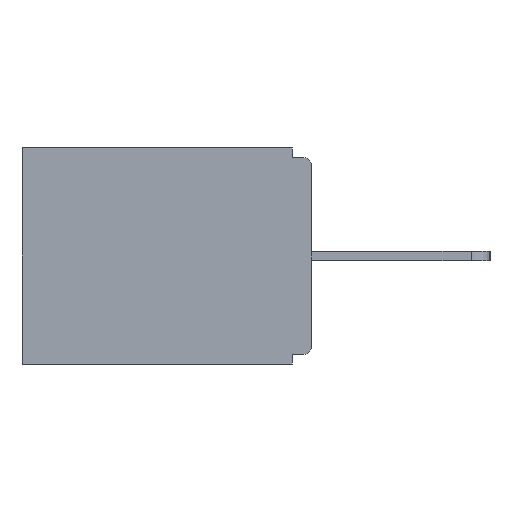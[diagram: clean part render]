
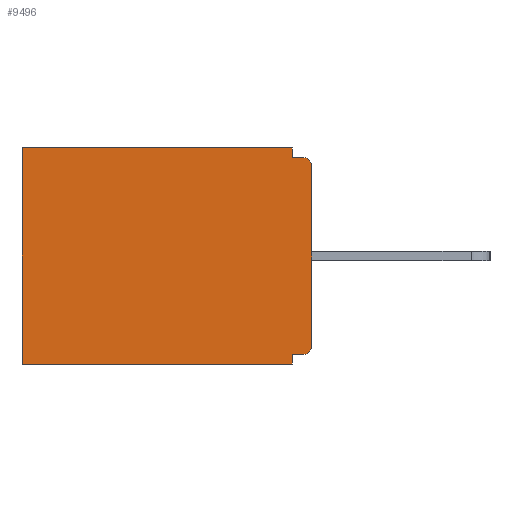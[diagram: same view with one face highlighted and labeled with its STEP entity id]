
A CAD part, left-side view. The second image highlights one B-rep face of the part: STEP entity #9496.
In plain terms, the highlighted planar face has unit normal (-1, 0, 0).
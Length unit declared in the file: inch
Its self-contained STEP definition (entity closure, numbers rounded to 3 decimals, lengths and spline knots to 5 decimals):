
#75 = DIRECTION ( 'NONE',  ( 0., 0., -1. ) ) ;
#274 = VECTOR ( 'NONE', #1478, 39.37008 ) ;
#306 = ORIENTED_EDGE ( 'NONE', *, *, #9947, .T. ) ;
#823 = CARTESIAN_POINT ( 'NONE',  ( 0.298, 0., -0.328 ) ) ;
#1016 = VECTOR ( 'NONE', #3457, 39.37008 ) ;
#1034 = FACE_OUTER_BOUND ( 'NONE', #3195, .T. ) ;
#1288 = EDGE_CURVE ( 'NONE', #5536, #6511, #2376, .T. ) ;
#1304 = CARTESIAN_POINT ( 'NONE',  ( 0.298, 0.031, -0.343 ) ) ;
#1478 = DIRECTION ( 'NONE',  ( 0., 1., 0. ) ) ;
#1483 = VECTOR ( 'NONE', #11408, 39.37008 ) ;
#1641 = CARTESIAN_POINT ( 'NONE',  ( 0.298, 0., -0.313 ) ) ;
#2095 = DIRECTION ( 'NONE',  ( 0., 1., 0. ) ) ;
#2112 = DIRECTION ( 'NONE',  ( -1., 0., 0. ) ) ;
#2376 = CIRCLE ( 'NONE', #4933, 0.015 ) ;
#2803 = LINE ( 'NONE', #11574, #1483 ) ;
#3195 = EDGE_LOOP ( 'NONE', ( #12392, #14324, #9235, #8560, #12011, #10672, #10726, #3994, #306, #14781 ) ) ;
#3457 = DIRECTION ( 'NONE',  ( 0., 0., -1. ) ) ;
#3497 = EDGE_CURVE ( 'NONE', #7280, #9284, #8838, .T. ) ;
#3994 = ORIENTED_EDGE ( 'NONE', *, *, #10938, .F. ) ;
#4331 = VECTOR ( 'NONE', #8509, 39.37008 ) ;
#4441 = VERTEX_POINT ( 'NONE', #13060 ) ;
#4472 = CARTESIAN_POINT ( 'NONE',  ( 0.298, 0.015, -0.015 ) ) ;
#4592 = DIRECTION ( 'NONE',  ( 0., 0., -1. ) ) ;
#4612 = AXIS2_PLACEMENT_3D ( 'NONE', #10541, #7449, #75 ) ;
#4714 = CARTESIAN_POINT ( 'NONE',  ( 0.298, 0.015, -0.328 ) ) ;
#4933 = AXIS2_PLACEMENT_3D ( 'NONE', #13312, #2112, #4592 ) ;
#5103 = CARTESIAN_POINT ( 'NONE',  ( 0.298, 0.46, 0. ) ) ;
#5301 = VECTOR ( 'NONE', #6205, 39.37008 ) ;
#5426 = CARTESIAN_POINT ( 'NONE',  ( 0.298, 0., -0.343 ) ) ;
#5442 = CARTESIAN_POINT ( 'NONE',  ( 0.298, 0.031, -0.015 ) ) ;
#5536 = VERTEX_POINT ( 'NONE', #6482 ) ;
#5719 = DIRECTION ( 'NONE',  ( 0., 0., -1. ) ) ;
#6205 = DIRECTION ( 'NONE',  ( 0., 0., -1. ) ) ;
#6429 = EDGE_CURVE ( 'NONE', #9284, #6511, #2803, .T. ) ;
#6482 = CARTESIAN_POINT ( 'NONE',  ( 0.298, 0., -0.03 ) ) ;
#6511 = VERTEX_POINT ( 'NONE', #4472 ) ;
#7197 = DIRECTION ( 'NONE',  ( -1., 0., 0. ) ) ;
#7280 = VERTEX_POINT ( 'NONE', #10399 ) ;
#7449 = DIRECTION ( 'NONE',  ( 1., 0., 0. ) ) ;
#8364 = VERTEX_POINT ( 'NONE', #11023 ) ;
#8509 = DIRECTION ( 'NONE',  ( 0., 1., 0. ) ) ;
#8541 = EDGE_CURVE ( 'NONE', #5536, #9723, #12091, .T. ) ;
#8555 = EDGE_CURVE ( 'NONE', #10921, #8364, #14481, .T. ) ;
#8560 = ORIENTED_EDGE ( 'NONE', *, *, #9128, .T. ) ;
#8838 = LINE ( 'NONE', #1304, #5301 ) ;
#9128 = EDGE_CURVE ( 'NONE', #7280, #14505, #14550, .T. ) ;
#9235 = ORIENTED_EDGE ( 'NONE', *, *, #3497, .F. ) ;
#9284 = VERTEX_POINT ( 'NONE', #5442 ) ;
#9311 = CARTESIAN_POINT ( 'NONE',  ( 0.298, 0.031, -0.328 ) ) ;
#9386 = CARTESIAN_POINT ( 'NONE',  ( 0.298, 0.031, -0.343 ) ) ;
#9496 = ADVANCED_FACE ( 'NONE', ( #1034 ), #11802, .F. ) ;
#9723 = VERTEX_POINT ( 'NONE', #1641 ) ;
#9734 = EDGE_CURVE ( 'NONE', #8364, #4441, #11245, .T. ) ;
#9850 = CARTESIAN_POINT ( 'NONE',  ( 0.298, 0., 0. ) ) ;
#9947 = EDGE_CURVE ( 'NONE', #10097, #9723, #13567, .T. ) ;
#10097 = VERTEX_POINT ( 'NONE', #4714 ) ;
#10399 = CARTESIAN_POINT ( 'NONE',  ( 0.298, 0.031, 0. ) ) ;
#10541 = CARTESIAN_POINT ( 'NONE',  ( 0.298, 0., 0. ) ) ;
#10672 = ORIENTED_EDGE ( 'NONE', *, *, #9734, .F. ) ;
#10701 = VECTOR ( 'NONE', #5719, 39.37008 ) ;
#10726 = ORIENTED_EDGE ( 'NONE', *, *, #8555, .F. ) ;
#10921 = VERTEX_POINT ( 'NONE', #9311 ) ;
#10938 = EDGE_CURVE ( 'NONE', #10097, #10921, #14164, .T. ) ;
#11023 = CARTESIAN_POINT ( 'NONE',  ( 0.298, 0.031, -0.343 ) ) ;
#11245 = LINE ( 'NONE', #5426, #274 ) ;
#11366 = DIRECTION ( 'NONE',  ( 0., 0., -1. ) ) ;
#11408 = DIRECTION ( 'NONE',  ( 0., -1., 0. ) ) ;
#11574 = CARTESIAN_POINT ( 'NONE',  ( 0.298, 0., -0.015 ) ) ;
#11802 = PLANE ( 'NONE',  #4612 ) ;
#11992 = VECTOR ( 'NONE', #11366, 39.37008 ) ;
#12011 = ORIENTED_EDGE ( 'NONE', *, *, #14855, .T. ) ;
#12023 = AXIS2_PLACEMENT_3D ( 'NONE', #14509, #7197, #13231 ) ;
#12091 = LINE ( 'NONE', #13133, #10701 ) ;
#12392 = ORIENTED_EDGE ( 'NONE', *, *, #1288, .T. ) ;
#12575 = LINE ( 'NONE', #13564, #11992 ) ;
#13060 = CARTESIAN_POINT ( 'NONE',  ( 0.298, 0.46, -0.343 ) ) ;
#13133 = CARTESIAN_POINT ( 'NONE',  ( 0.298, 0., 0. ) ) ;
#13231 = DIRECTION ( 'NONE',  ( 0., 0., -1. ) ) ;
#13312 = CARTESIAN_POINT ( 'NONE',  ( 0.298, 0.015, -0.03 ) ) ;
#13564 = CARTESIAN_POINT ( 'NONE',  ( 0.298, 0.46, 0. ) ) ;
#13567 = CIRCLE ( 'NONE', #12023, 0.015 ) ;
#14164 = LINE ( 'NONE', #823, #14858 ) ;
#14324 = ORIENTED_EDGE ( 'NONE', *, *, #6429, .F. ) ;
#14481 = LINE ( 'NONE', #9386, #1016 ) ;
#14505 = VERTEX_POINT ( 'NONE', #5103 ) ;
#14509 = CARTESIAN_POINT ( 'NONE',  ( 0.298, 0.015, -0.313 ) ) ;
#14550 = LINE ( 'NONE', #9850, #4331 ) ;
#14781 = ORIENTED_EDGE ( 'NONE', *, *, #8541, .F. ) ;
#14855 = EDGE_CURVE ( 'NONE', #14505, #4441, #12575, .T. ) ;
#14858 = VECTOR ( 'NONE', #2095, 39.37008 ) ;
